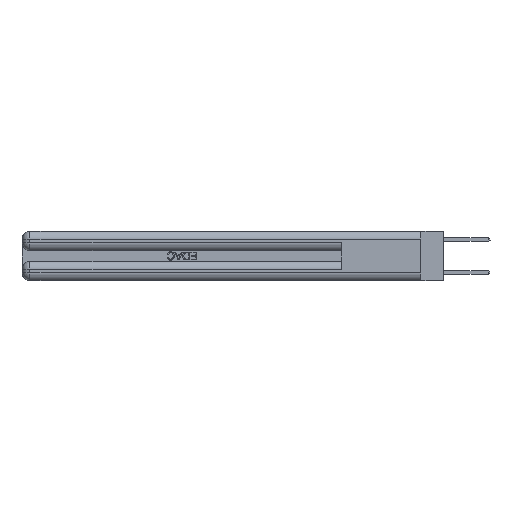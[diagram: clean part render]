
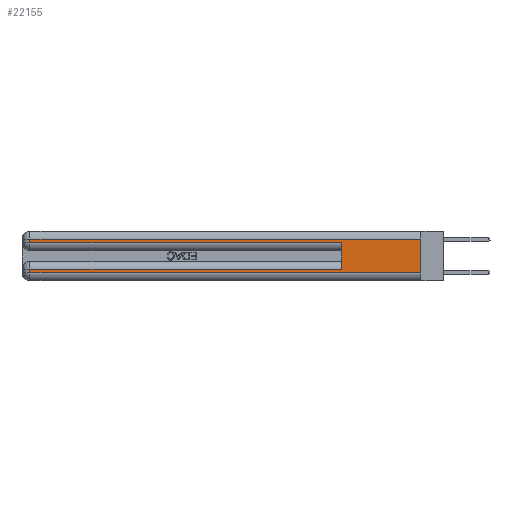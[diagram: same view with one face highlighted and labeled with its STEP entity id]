
A CAD part, left-side view. The second image highlights one B-rep face of the part: STEP entity #22155.
In plain terms, the highlighted planar face has unit normal (-1, 0, 0).
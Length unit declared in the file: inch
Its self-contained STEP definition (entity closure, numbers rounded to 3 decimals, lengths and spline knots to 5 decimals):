
#206 = ORIENTED_EDGE ( 'NONE', *, *, #14579, .T. ) ;
#291 = CARTESIAN_POINT ( 'NONE',  ( 0., 2.94, 0.085 ) ) ;
#432 = ORIENTED_EDGE ( 'NONE', *, *, #12627, .F. ) ;
#479 = VERTEX_POINT ( 'NONE', #6532 ) ;
#548 = DIRECTION ( 'NONE',  ( 0., -1., 0. ) ) ;
#1051 = DIRECTION ( 'NONE',  ( 0., 0., -1. ) ) ;
#1286 = VERTEX_POINT ( 'NONE', #24422 ) ;
#1400 = DIRECTION ( 'NONE',  ( 0., 0., -1. ) ) ;
#1485 = ORIENTED_EDGE ( 'NONE', *, *, #12092, .T. ) ;
#1869 = EDGE_CURVE ( 'NONE', #14446, #479, #24590, .T. ) ;
#1941 = DIRECTION ( 'NONE',  ( 0., 0., -1. ) ) ;
#2526 = LINE ( 'NONE', #15294, #14892 ) ;
#3868 = VECTOR ( 'NONE', #1051, 39.37008 ) ;
#4000 = VECTOR ( 'NONE', #7971, 39.37008 ) ;
#4781 = LINE ( 'NONE', #5496, #4000 ) ;
#5496 = CARTESIAN_POINT ( 'NONE',  ( 0., 0., 0.06 ) ) ;
#5549 = CARTESIAN_POINT ( 'NONE',  ( 0., 0., 0.285 ) ) ;
#5600 = VERTEX_POINT ( 'NONE', #11914 ) ;
#5861 = ORIENTED_EDGE ( 'NONE', *, *, #19645, .T. ) ;
#6438 = LINE ( 'NONE', #21744, #31680 ) ;
#6499 = VERTEX_POINT ( 'NONE', #291 ) ;
#6532 = CARTESIAN_POINT ( 'NONE',  ( 0., 0., 0.06 ) ) ;
#7225 = ORIENTED_EDGE ( 'NONE', *, *, #13303, .T. ) ;
#7971 = DIRECTION ( 'NONE',  ( 0., -1., 0. ) ) ;
#11914 = CARTESIAN_POINT ( 'NONE',  ( 0., 0.6, 0.085 ) ) ;
#12092 = EDGE_CURVE ( 'NONE', #29526, #1286, #15747, .T. ) ;
#12627 = EDGE_CURVE ( 'NONE', #5600, #21802, #6438, .T. ) ;
#12965 = CARTESIAN_POINT ( 'NONE',  ( 0., 0.6, 0.285 ) ) ;
#13303 = EDGE_CURVE ( 'NONE', #5600, #6499, #2526, .T. ) ;
#13379 = CARTESIAN_POINT ( 'NONE',  ( 0., 2.94, 0.37 ) ) ;
#13750 = FACE_OUTER_BOUND ( 'NONE', #31329, .T. ) ;
#14350 = ORIENTED_EDGE ( 'NONE', *, *, #16459, .T. ) ;
#14446 = VERTEX_POINT ( 'NONE', #16464 ) ;
#14579 = EDGE_CURVE ( 'NONE', #18732, #479, #4781, .T. ) ;
#14892 = VECTOR ( 'NONE', #17760, 39.37008 ) ;
#15222 = CARTESIAN_POINT ( 'NONE',  ( 0., 2.94, 0.06 ) ) ;
#15294 = CARTESIAN_POINT ( 'NONE',  ( 0., 0., 0.085 ) ) ;
#15747 = LINE ( 'NONE', #31734, #27192 ) ;
#15781 = LINE ( 'NONE', #31400, #28756 ) ;
#16168 = DIRECTION ( 'NONE',  ( 1., 0., 0. ) ) ;
#16459 = EDGE_CURVE ( 'NONE', #1286, #21802, #18508, .T. ) ;
#16464 = CARTESIAN_POINT ( 'NONE',  ( 0., 0., 0.31 ) ) ;
#16803 = DIRECTION ( 'NONE',  ( 0., 1., 0. ) ) ;
#17172 = DIRECTION ( 'NONE',  ( 0., 0., -1. ) ) ;
#17760 = DIRECTION ( 'NONE',  ( 0., 1., 0. ) ) ;
#18230 = CARTESIAN_POINT ( 'NONE',  ( 0., 2.94, 0.31 ) ) ;
#18508 = LINE ( 'NONE', #5549, #25007 ) ;
#18732 = VERTEX_POINT ( 'NONE', #15222 ) ;
#18861 = EDGE_CURVE ( 'NONE', #6499, #18732, #29943, .T. ) ;
#19645 = EDGE_CURVE ( 'NONE', #14446, #29526, #15781, .T. ) ;
#21744 = CARTESIAN_POINT ( 'NONE',  ( 0., 0.6, 0.145 ) ) ;
#21802 = VERTEX_POINT ( 'NONE', #12965 ) ;
#22155 = ADVANCED_FACE ( 'NONE', ( #13750 ), #30774, .F. ) ;
#24190 = DIRECTION ( 'NONE',  ( 0., 0., 1. ) ) ;
#24422 = CARTESIAN_POINT ( 'NONE',  ( 0., 2.94, 0.285 ) ) ;
#24590 = LINE ( 'NONE', #31285, #29543 ) ;
#25007 = VECTOR ( 'NONE', #548, 39.37008 ) ;
#25896 = CARTESIAN_POINT ( 'NONE',  ( 0., 0., 0.37 ) ) ;
#26361 = ORIENTED_EDGE ( 'NONE', *, *, #18861, .T. ) ;
#27192 = VECTOR ( 'NONE', #17172, 39.37008 ) ;
#28756 = VECTOR ( 'NONE', #16803, 39.37008 ) ;
#29127 = ORIENTED_EDGE ( 'NONE', *, *, #1869, .F. ) ;
#29510 = AXIS2_PLACEMENT_3D ( 'NONE', #25896, #16168, #1400 ) ;
#29526 = VERTEX_POINT ( 'NONE', #18230 ) ;
#29543 = VECTOR ( 'NONE', #1941, 39.37008 ) ;
#29943 = LINE ( 'NONE', #13379, #3868 ) ;
#30774 = PLANE ( 'NONE',  #29510 ) ;
#31285 = CARTESIAN_POINT ( 'NONE',  ( 0., 0., 0.37 ) ) ;
#31329 = EDGE_LOOP ( 'NONE', ( #29127, #5861, #1485, #14350, #432, #7225, #26361, #206 ) ) ;
#31400 = CARTESIAN_POINT ( 'NONE',  ( 0., 0., 0.31 ) ) ;
#31680 = VECTOR ( 'NONE', #24190, 39.37008 ) ;
#31734 = CARTESIAN_POINT ( 'NONE',  ( 0., 2.94, 0.37 ) ) ;
